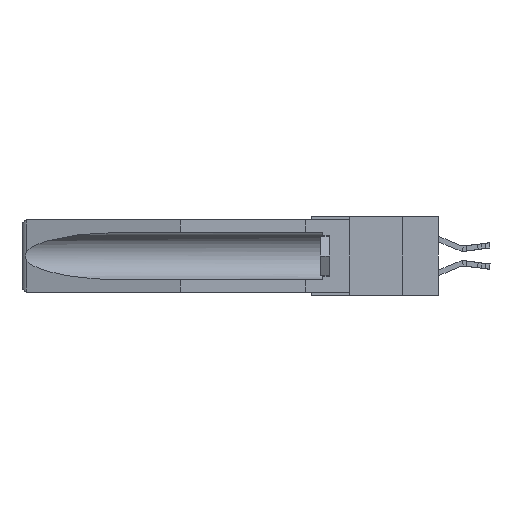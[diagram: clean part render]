
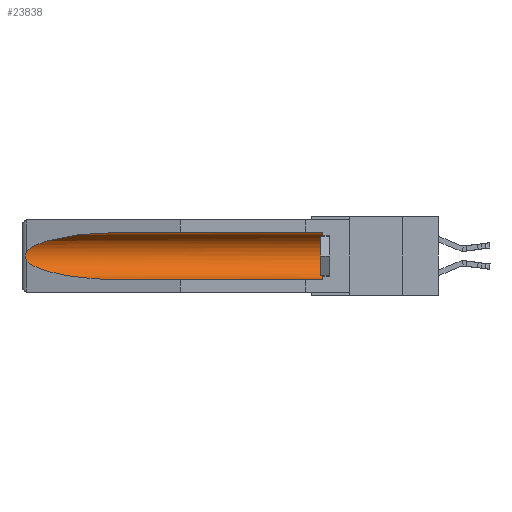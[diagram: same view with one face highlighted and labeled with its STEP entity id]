
A CAD part, left-side view. The second image highlights one B-rep face of the part: STEP entity #23838.
In plain terms, the highlighted cylindrical face has radius 2.857 mm (diameter 5.715 mm), a partial arc.
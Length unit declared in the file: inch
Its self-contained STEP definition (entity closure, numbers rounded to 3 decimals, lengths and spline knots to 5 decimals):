
#224 = CARTESIAN_POINT ( 'NONE',  ( 0.26655, 1.53094, -0.18657 ) ) ;
#454 = CARTESIAN_POINT ( 'NONE',  ( 0.2673, 1.5327, -0.16383 ) ) ;
#1002 = EDGE_CURVE ( 'NONE', #13029, #21000, #14421, .T. ) ;
#1465 = EDGE_CURVE ( 'NONE', #34389, #23359, #27640, .T. ) ;
#2101 = EDGE_CURVE ( 'NONE', #4194, #34389, #22904, .T. ) ;
#2545 = CARTESIAN_POINT ( 'NONE',  ( 0.155, 1.07973, -0.059 ) ) ;
#3168 = CARTESIAN_POINT ( 'NONE',  ( 0.2675, 1.53308, -0.17534 ) ) ;
#4194 = VERTEX_POINT ( 'NONE', #6633 ) ;
#5202 = DIRECTION ( 'NONE',  ( 0., 0., 1. ) ) ;
#5802 = AXIS2_PLACEMENT_3D ( 'NONE', #11377, #19473, #32974 ) ;
#6633 = CARTESIAN_POINT ( 'NONE',  ( 0.26537, 1.52718, -0.14972 ) ) ;
#8377 = CARTESIAN_POINT ( 'NONE',  ( 0.26597, 1.52961, -0.15275 ) ) ;
#11377 = CARTESIAN_POINT ( 'NONE',  ( 0.155, -0.30754, -0.1715 ) ) ;
#11713 = VECTOR ( 'NONE', #26326, 39.37008 ) ;
#11913 =( BOUNDED_CURVE ( )  B_SPLINE_CURVE ( 3, ( #22392, #17207, #14300, #27921 ),
 .UNSPECIFIED., .F., .T. ) 
 B_SPLINE_CURVE_WITH_KNOTS ( ( 4, 4 ),
 ( 4.71239, 6.08839 ),
 .UNSPECIFIED. ) 
 CURVE ( )  GEOMETRIC_REPRESENTATION_ITEM ( )  RATIONAL_B_SPLINE_CURVE ( ( 1., 0.848, 0.848, 1. ) ) 
 REPRESENTATION_ITEM ( '' )  );
#12225 = CYLINDRICAL_SURFACE ( 'NONE', #5802, 0.1125 ) ;
#12499 = CARTESIAN_POINT ( 'NONE',  ( 0.26537, 1.52718, -0.19328 ) ) ;
#12679 = CARTESIAN_POINT ( 'NONE',  ( 0.155, -0.30754, -0.059 ) ) ;
#13029 = VERTEX_POINT ( 'NONE', #32116 ) ;
#13527 = CARTESIAN_POINT ( 'NONE',  ( 0.26537, 1.52718, -0.19328 ) ) ;
#13917 = FACE_OUTER_BOUND ( 'NONE', #24593, .T. ) ;
#14300 = CARTESIAN_POINT ( 'NONE',  ( 0.25451, 1.48313, -0.09465 ) ) ;
#14421 = CIRCLE ( 'NONE', #16786, 0.1125 ) ;
#15040 = CARTESIAN_POINT ( 'NONE',  ( 0.155, 1.07973, -0.284 ) ) ;
#16786 = AXIS2_PLACEMENT_3D ( 'NONE', #21644, #18827, #5202 ) ;
#16968 = VERTEX_POINT ( 'NONE', #2545 ) ;
#17207 = CARTESIAN_POINT ( 'NONE',  ( 0.21114, 1.30732, -0.059 ) ) ;
#18749 = EDGE_CURVE ( 'NONE', #16968, #4194, #11913, .T. ) ;
#18827 = DIRECTION ( 'NONE',  ( 0., -1., 0. ) ) ;
#19082 = CARTESIAN_POINT ( 'NONE',  ( 0.155, 1.07973, -0.284 ) ) ;
#19473 = DIRECTION ( 'NONE',  ( 0., 1., 0. ) ) ;
#21000 = VERTEX_POINT ( 'NONE', #34486 ) ;
#21416 = DIRECTION ( 'NONE',  ( 0., 1., 0. ) ) ;
#21634 = ORIENTED_EDGE ( 'NONE', *, *, #18749, .T. ) ;
#21639 = CARTESIAN_POINT ( 'NONE',  ( 0.26654, 1.53092, -0.15636 ) ) ;
#21644 = CARTESIAN_POINT ( 'NONE',  ( 0.155, 0.126, -0.1715 ) ) ;
#21862 = CARTESIAN_POINT ( 'NONE',  ( 0.26597, 1.5296, -0.19026 ) ) ;
#21988 = CARTESIAN_POINT ( 'NONE',  ( 0.2673, 1.53269, -0.17917 ) ) ;
#22392 = CARTESIAN_POINT ( 'NONE',  ( 0.155, 1.07973, -0.059 ) ) ;
#22904 = B_SPLINE_CURVE_WITH_KNOTS ( 'NONE', 3,
 ( #32666, #8377, #21639, #454, #32426, #3168, #21988, #224, #21862, #13527 ),
 .UNSPECIFIED., .F., .F.,
 ( 4, 2, 2, 2, 4 ),
 ( 0., 0.00029, 0.00058, 0.00087, 0.00117 ),
 .UNSPECIFIED. ) ;
#23258 = CARTESIAN_POINT ( 'NONE',  ( 0.21114, 1.30732, -0.284 ) ) ;
#23359 = VERTEX_POINT ( 'NONE', #19082 ) ;
#23493 = LINE ( 'NONE', #12679, #11713 ) ;
#23838 = ADVANCED_FACE ( 'NONE', ( #13917 ), #12225, .F. ) ;
#24120 = LINE ( 'NONE', #29499, #28718 ) ;
#24593 = EDGE_LOOP ( 'NONE', ( #21634, #26108, #27576, #32428, #27783, #32844 ) ) ;
#25717 = CARTESIAN_POINT ( 'NONE',  ( 0.26537, 1.52718, -0.19328 ) ) ;
#25968 = CARTESIAN_POINT ( 'NONE',  ( 0.25451, 1.48313, -0.24835 ) ) ;
#26108 = ORIENTED_EDGE ( 'NONE', *, *, #2101, .T. ) ;
#26326 = DIRECTION ( 'NONE',  ( 0., 1., 0. ) ) ;
#27576 = ORIENTED_EDGE ( 'NONE', *, *, #1465, .T. ) ;
#27640 =( BOUNDED_CURVE ( )  B_SPLINE_CURVE ( 3, ( #25717, #25968, #23258, #15040 ),
 .UNSPECIFIED., .F., .T. ) 
 B_SPLINE_CURVE_WITH_KNOTS ( ( 4, 4 ),
 ( 0.1948, 1.5708 ),
 .UNSPECIFIED. ) 
 CURVE ( )  GEOMETRIC_REPRESENTATION_ITEM ( )  RATIONAL_B_SPLINE_CURVE ( ( 1., 0.848, 0.848, 1. ) ) 
 REPRESENTATION_ITEM ( '' )  );
#27783 = ORIENTED_EDGE ( 'NONE', *, *, #1002, .T. ) ;
#27921 = CARTESIAN_POINT ( 'NONE',  ( 0.26537, 1.52718, -0.14972 ) ) ;
#28718 = VECTOR ( 'NONE', #21416, 39.37008 ) ;
#29499 = CARTESIAN_POINT ( 'NONE',  ( 0.155, -0.30754, -0.284 ) ) ;
#30695 = EDGE_CURVE ( 'NONE', #21000, #16968, #23493, .T. ) ;
#32116 = CARTESIAN_POINT ( 'NONE',  ( 0.155, 0.126, -0.284 ) ) ;
#32426 = CARTESIAN_POINT ( 'NONE',  ( 0.2675, 1.53308, -0.16763 ) ) ;
#32428 = ORIENTED_EDGE ( 'NONE', *, *, #34532, .F. ) ;
#32666 = CARTESIAN_POINT ( 'NONE',  ( 0.26537, 1.52718, -0.14972 ) ) ;
#32844 = ORIENTED_EDGE ( 'NONE', *, *, #30695, .T. ) ;
#32974 = DIRECTION ( 'NONE',  ( 0., 0., 1. ) ) ;
#34389 = VERTEX_POINT ( 'NONE', #12499 ) ;
#34486 = CARTESIAN_POINT ( 'NONE',  ( 0.155, 0.126, -0.059 ) ) ;
#34532 = EDGE_CURVE ( 'NONE', #13029, #23359, #24120, .T. ) ;
